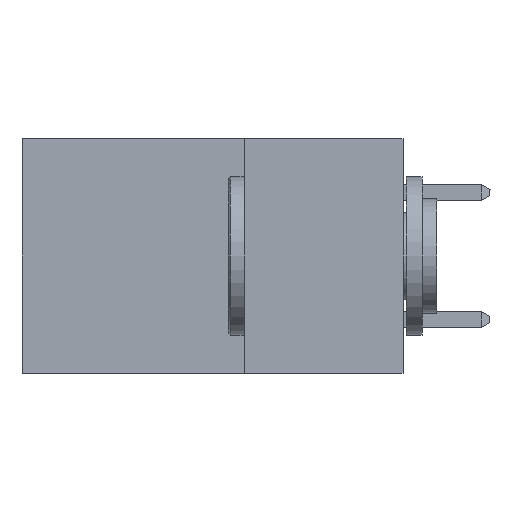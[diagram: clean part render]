
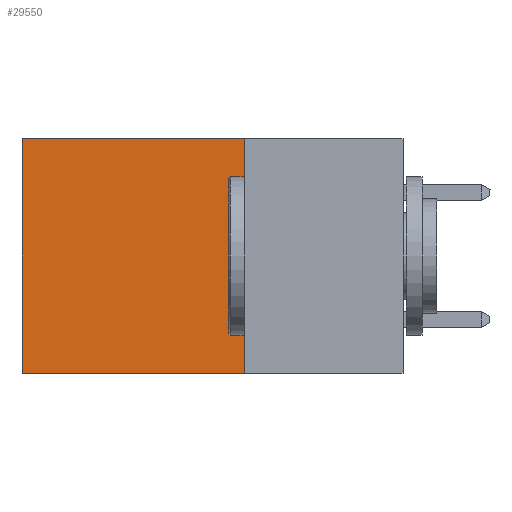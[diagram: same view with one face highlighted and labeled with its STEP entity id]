
A CAD part, left-side view. The second image highlights one B-rep face of the part: STEP entity #29550.
In plain terms, the highlighted planar face has unit normal (-1, 0, 0).
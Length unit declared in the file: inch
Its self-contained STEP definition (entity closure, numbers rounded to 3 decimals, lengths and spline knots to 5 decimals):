
#1332 = DIRECTION ( 'NONE',  ( 0., 0., -1. ) ) ;
#1733 = AXIS2_PLACEMENT_3D ( 'NONE', #13189, #30109, #15647 ) ;
#5887 = VECTOR ( 'NONE', #15368, 39.37008 ) ;
#6220 = CARTESIAN_POINT ( 'NONE',  ( 0.2875, 0.6, -0.37 ) ) ;
#10013 = CARTESIAN_POINT ( 'NONE',  ( 0.2875, 0.25, 0. ) ) ;
#10533 = VERTEX_POINT ( 'NONE', #25488 ) ;
#11225 = VERTEX_POINT ( 'NONE', #6220 ) ;
#12208 = CARTESIAN_POINT ( 'NONE',  ( 0.2875, 0.25, -0.37 ) ) ;
#12274 = CARTESIAN_POINT ( 'NONE',  ( 0.2875, 0.25, 0. ) ) ;
#13086 = PLANE ( 'NONE',  #1733 ) ;
#13189 = CARTESIAN_POINT ( 'NONE',  ( 0.2875, 0.25, 0. ) ) ;
#13612 = ORIENTED_EDGE ( 'NONE', *, *, #15790, .T. ) ;
#14667 = DIRECTION ( 'NONE',  ( 0., 1., 0. ) ) ;
#14913 = CARTESIAN_POINT ( 'NONE',  ( 0.2875, 0.25, -0.37 ) ) ;
#15368 = DIRECTION ( 'NONE',  ( 0., 0., -1. ) ) ;
#15647 = DIRECTION ( 'NONE',  ( 0., 0., -1. ) ) ;
#15790 = EDGE_CURVE ( 'NONE', #10533, #11225, #24293, .T. ) ;
#17852 = VECTOR ( 'NONE', #1332, 39.37008 ) ;
#18410 = VECTOR ( 'NONE', #14667, 39.37008 ) ;
#18855 = LINE ( 'NONE', #20246, #5887 ) ;
#20246 = CARTESIAN_POINT ( 'NONE',  ( 0.2875, 0.25, 0. ) ) ;
#20941 = CARTESIAN_POINT ( 'NONE',  ( 0.2875, 0.6, 0. ) ) ;
#21283 = VECTOR ( 'NONE', #21909, 39.37008 ) ;
#21909 = DIRECTION ( 'NONE',  ( 0., 1., 0. ) ) ;
#22594 = FACE_OUTER_BOUND ( 'NONE', #26465, .T. ) ;
#23322 = LINE ( 'NONE', #12208, #18410 ) ;
#23545 = ORIENTED_EDGE ( 'NONE', *, *, #28849, .F. ) ;
#24293 = LINE ( 'NONE', #20941, #17852 ) ;
#24612 = EDGE_CURVE ( 'NONE', #27381, #10533, #28456, .T. ) ;
#25488 = CARTESIAN_POINT ( 'NONE',  ( 0.2875, 0.6, 0. ) ) ;
#26465 = EDGE_LOOP ( 'NONE', ( #13612, #29521, #23545, #31670 ) ) ;
#27381 = VERTEX_POINT ( 'NONE', #10013 ) ;
#28456 = LINE ( 'NONE', #12274, #21283 ) ;
#28849 = EDGE_CURVE ( 'NONE', #27381, #29382, #18855, .T. ) ;
#29382 = VERTEX_POINT ( 'NONE', #14913 ) ;
#29521 = ORIENTED_EDGE ( 'NONE', *, *, #29977, .F. ) ;
#29550 = ADVANCED_FACE ( 'NONE', ( #22594 ), #13086, .F. ) ;
#29977 = EDGE_CURVE ( 'NONE', #29382, #11225, #23322, .T. ) ;
#30109 = DIRECTION ( 'NONE',  ( 1., 0., 0. ) ) ;
#31670 = ORIENTED_EDGE ( 'NONE', *, *, #24612, .T. ) ;
